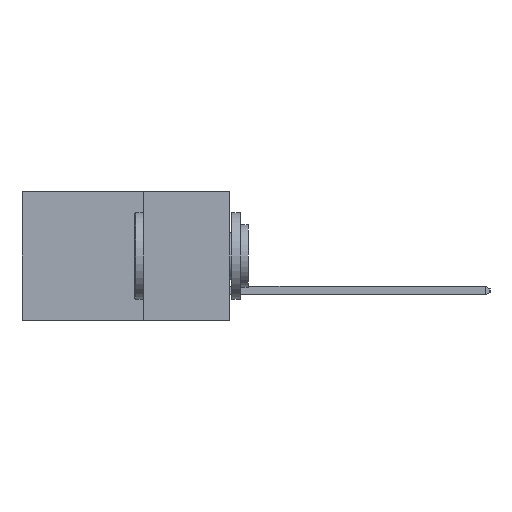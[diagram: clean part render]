
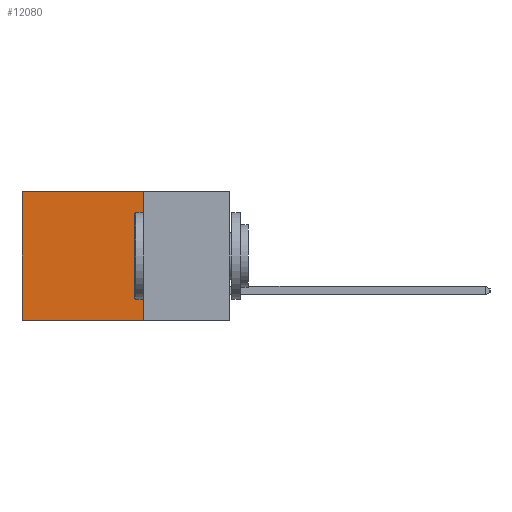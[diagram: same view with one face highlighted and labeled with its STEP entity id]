
A CAD part, left-side view. The second image highlights one B-rep face of the part: STEP entity #12080.
In plain terms, the highlighted planar face has unit normal (-1, 0, 0).
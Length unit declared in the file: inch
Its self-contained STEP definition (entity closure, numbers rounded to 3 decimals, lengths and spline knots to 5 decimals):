
#89 = CARTESIAN_POINT ( 'NONE',  ( 0.298, 0.6, 0. ) ) ;
#1516 = PLANE ( 'NONE',  #26782 ) ;
#2399 = CARTESIAN_POINT ( 'NONE',  ( 0.298, 0.6, 0. ) ) ;
#2945 = EDGE_CURVE ( 'NONE', #27763, #17569, #17827, .T. ) ;
#3940 = ORIENTED_EDGE ( 'NONE', *, *, #2945, .F. ) ;
#4524 = VECTOR ( 'NONE', #13337, 39.37008 ) ;
#4574 = EDGE_CURVE ( 'NONE', #25063, #27763, #14258, .T. ) ;
#5478 = CARTESIAN_POINT ( 'NONE',  ( 0.298, 0.25, -0.37 ) ) ;
#5497 = LINE ( 'NONE', #89, #17338 ) ;
#5536 = CARTESIAN_POINT ( 'NONE',  ( 0.298, 0.25, -0.37 ) ) ;
#6279 = DIRECTION ( 'NONE',  ( 0., 0., -1. ) ) ;
#6319 = EDGE_LOOP ( 'NONE', ( #27151, #3940, #20981, #27664 ) ) ;
#7741 = DIRECTION ( 'NONE',  ( 0., 0., -1. ) ) ;
#7785 = CARTESIAN_POINT ( 'NONE',  ( 0.298, 0.25, 0. ) ) ;
#8742 = VECTOR ( 'NONE', #7741, 39.37008 ) ;
#9135 = CARTESIAN_POINT ( 'NONE',  ( 0.298, 0.6, -0.37 ) ) ;
#10614 = VERTEX_POINT ( 'NONE', #2399 ) ;
#12080 = ADVANCED_FACE ( 'NONE', ( #27102 ), #1516, .F. ) ;
#12189 = VECTOR ( 'NONE', #13505, 39.37008 ) ;
#13337 = DIRECTION ( 'NONE',  ( 0., 1., 0. ) ) ;
#13505 = DIRECTION ( 'NONE',  ( 0., 1., 0. ) ) ;
#14258 = LINE ( 'NONE', #7785, #8742 ) ;
#15818 = EDGE_CURVE ( 'NONE', #10614, #17569, #5497, .T. ) ;
#15845 = CARTESIAN_POINT ( 'NONE',  ( 0.298, 0.25, 0. ) ) ;
#16615 = DIRECTION ( 'NONE',  ( 0., 0., -1. ) ) ;
#17338 = VECTOR ( 'NONE', #16615, 39.37008 ) ;
#17569 = VERTEX_POINT ( 'NONE', #9135 ) ;
#17827 = LINE ( 'NONE', #5536, #4524 ) ;
#18014 = CARTESIAN_POINT ( 'NONE',  ( 0.298, 0.25, 0. ) ) ;
#18412 = LINE ( 'NONE', #15845, #12189 ) ;
#20319 = EDGE_CURVE ( 'NONE', #25063, #10614, #18412, .T. ) ;
#20408 = DIRECTION ( 'NONE',  ( 1., 0., 0. ) ) ;
#20981 = ORIENTED_EDGE ( 'NONE', *, *, #4574, .F. ) ;
#24643 = CARTESIAN_POINT ( 'NONE',  ( 0.298, 0.25, 0. ) ) ;
#25063 = VERTEX_POINT ( 'NONE', #24643 ) ;
#26782 = AXIS2_PLACEMENT_3D ( 'NONE', #18014, #20408, #6279 ) ;
#27102 = FACE_OUTER_BOUND ( 'NONE', #6319, .T. ) ;
#27151 = ORIENTED_EDGE ( 'NONE', *, *, #15818, .T. ) ;
#27664 = ORIENTED_EDGE ( 'NONE', *, *, #20319, .T. ) ;
#27763 = VERTEX_POINT ( 'NONE', #5478 ) ;
